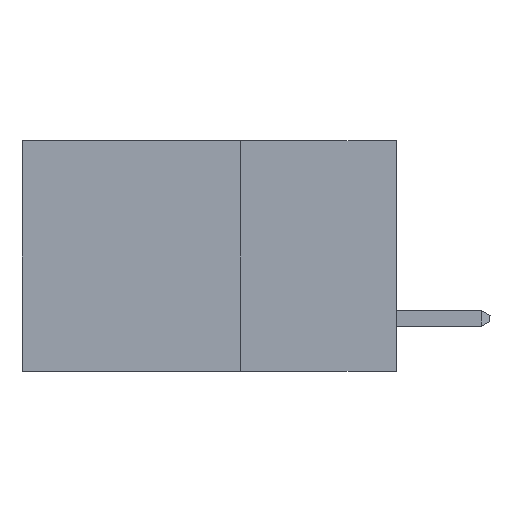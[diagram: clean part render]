
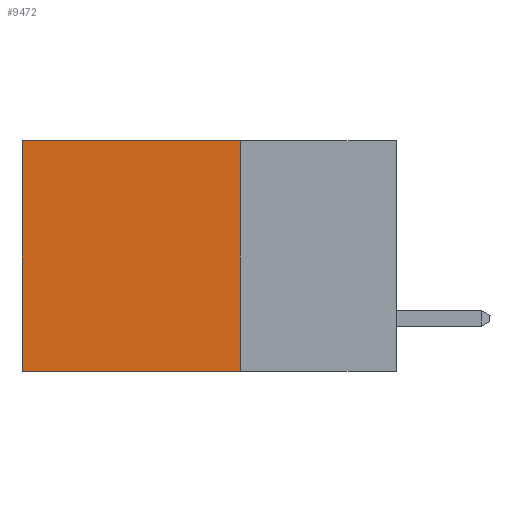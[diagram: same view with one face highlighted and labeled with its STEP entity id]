
A CAD part, left-side view. The second image highlights one B-rep face of the part: STEP entity #9472.
In plain terms, the highlighted planar face has unit normal (-1, 0, 0).
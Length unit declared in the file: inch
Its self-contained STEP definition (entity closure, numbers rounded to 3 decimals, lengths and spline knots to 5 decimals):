
#119 = LINE ( 'NONE', #1724, #6236 ) ;
#151 = CARTESIAN_POINT ( 'NONE',  ( 0.2615, 0.25, 0. ) ) ;
#418 = LINE ( 'NONE', #2155, #4200 ) ;
#722 = VECTOR ( 'NONE', #801, 39.37008 ) ;
#801 = DIRECTION ( 'NONE',  ( 0., 0., -1. ) ) ;
#953 = VERTEX_POINT ( 'NONE', #10376 ) ;
#1596 = FACE_OUTER_BOUND ( 'NONE', #3882, .T. ) ;
#1724 = CARTESIAN_POINT ( 'NONE',  ( 0.2615, 0.25, -0.37 ) ) ;
#2155 = CARTESIAN_POINT ( 'NONE',  ( 0.2615, 0.25, 0. ) ) ;
#2221 = ORIENTED_EDGE ( 'NONE', *, *, #6691, .F. ) ;
#3101 = DIRECTION ( 'NONE',  ( 0., 0., -1. ) ) ;
#3882 = EDGE_LOOP ( 'NONE', ( #8428, #9469, #2221, #10516 ) ) ;
#4200 = VECTOR ( 'NONE', #8629, 39.37008 ) ;
#4494 = EDGE_CURVE ( 'NONE', #953, #9386, #6628, .T. ) ;
#4663 = DIRECTION ( 'NONE',  ( 0., 1., 0. ) ) ;
#4714 = AXIS2_PLACEMENT_3D ( 'NONE', #5619, #4848, #3101 ) ;
#4848 = DIRECTION ( 'NONE',  ( 1., 0., 0. ) ) ;
#5557 = VECTOR ( 'NONE', #4663, 39.37008 ) ;
#5619 = CARTESIAN_POINT ( 'NONE',  ( 0.2615, 0.25, -0.37 ) ) ;
#5674 = CARTESIAN_POINT ( 'NONE',  ( 0.2615, 0.6, -0.37 ) ) ;
#6153 = CARTESIAN_POINT ( 'NONE',  ( 0.2615, 0.25, -0.37 ) ) ;
#6236 = VECTOR ( 'NONE', #8323, 39.37008 ) ;
#6508 = EDGE_CURVE ( 'NONE', #9071, #9386, #10273, .T. ) ;
#6628 = LINE ( 'NONE', #5674, #722 ) ;
#6691 = EDGE_CURVE ( 'NONE', #7567, #9071, #119, .T. ) ;
#7567 = VERTEX_POINT ( 'NONE', #151 ) ;
#8323 = DIRECTION ( 'NONE',  ( 0., 0., -1. ) ) ;
#8428 = ORIENTED_EDGE ( 'NONE', *, *, #4494, .T. ) ;
#8629 = DIRECTION ( 'NONE',  ( 0., 1., 0. ) ) ;
#9002 = EDGE_CURVE ( 'NONE', #7567, #953, #418, .T. ) ;
#9071 = VERTEX_POINT ( 'NONE', #6153 ) ;
#9386 = VERTEX_POINT ( 'NONE', #10454 ) ;
#9469 = ORIENTED_EDGE ( 'NONE', *, *, #6508, .F. ) ;
#9472 = ADVANCED_FACE ( 'NONE', ( #1596 ), #9570, .F. ) ;
#9570 = PLANE ( 'NONE',  #4714 ) ;
#10273 = LINE ( 'NONE', #10474, #5557 ) ;
#10376 = CARTESIAN_POINT ( 'NONE',  ( 0.2615, 0.6, 0. ) ) ;
#10454 = CARTESIAN_POINT ( 'NONE',  ( 0.2615, 0.6, -0.37 ) ) ;
#10474 = CARTESIAN_POINT ( 'NONE',  ( 0.2615, 0.25, -0.37 ) ) ;
#10516 = ORIENTED_EDGE ( 'NONE', *, *, #9002, .T. ) ;
